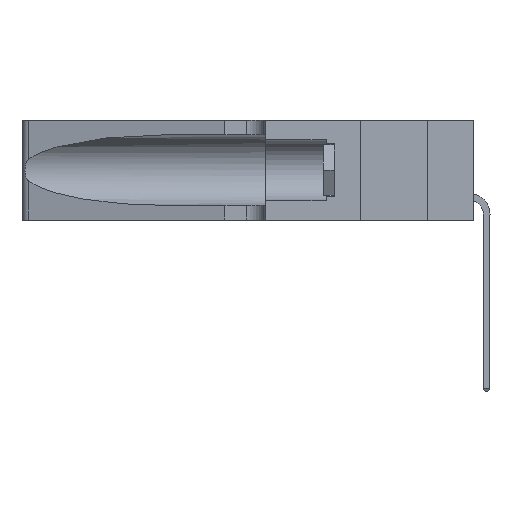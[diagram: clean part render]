
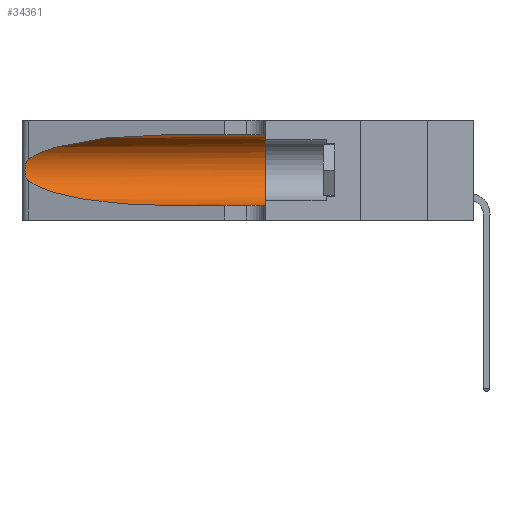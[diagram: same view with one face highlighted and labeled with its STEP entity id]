
A CAD part, left-side view. The second image highlights one B-rep face of the part: STEP entity #34361.
In plain terms, the highlighted cylindrical face has radius 3.308 mm (diameter 6.617 mm), a partial arc.
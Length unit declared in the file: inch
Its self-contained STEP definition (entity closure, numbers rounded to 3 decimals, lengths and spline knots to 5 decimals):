
#436 = CARTESIAN_POINT ( 'NONE',  ( 0.2373, 1.15595, 0.28018 ) ) ;
#444 =( BOUNDED_CURVE ( )  B_SPLINE_CURVE ( 3, ( #21980, #5683, #436, #24689 ),
 .UNSPECIFIED., .F., .F. ) 
 B_SPLINE_CURVE_WITH_KNOTS ( ( 4, 4 ),
 ( 1.5708, 2.84003 ),
 .UNSPECIFIED. ) 
 CURVE ( )  GEOMETRIC_REPRESENTATION_ITEM ( )  RATIONAL_B_SPLINE_CURVE ( ( 1., 0.87, 0.87, 1. ) ) 
 REPRESENTATION_ITEM ( '' )  );
#548 = ORIENTED_EDGE ( 'NONE', *, *, #11489, .F. ) ;
#1905 = CARTESIAN_POINT ( 'NONE',  ( 0.26018, 1.23835, 0.19895 ) ) ;
#3165 = VECTOR ( 'NONE', #34312, 39.37008 ) ;
#5121 = CARTESIAN_POINT ( 'NONE',  ( 0.25639, 1.23186, 0.15144 ) ) ;
#5570 = VERTEX_POINT ( 'NONE', #26565 ) ;
#5683 = CARTESIAN_POINT ( 'NONE',  ( 0.18966, 0.96281, 0.31525 ) ) ;
#6237 = CARTESIAN_POINT ( 'NONE',  ( 0.1305, 0.35, 0.31525 ) ) ;
#6379 = CARTESIAN_POINT ( 'NONE',  ( 0.18966, 0.96281, 0.05475 ) ) ;
#7819 = LINE ( 'NONE', #33601, #3165 ) ;
#7824 = EDGE_LOOP ( 'NONE', ( #22630, #31038, #19083, #35219, #32753, #548 ) ) ;
#8056 = CYLINDRICAL_SURFACE ( 'NONE', #14694, 0.13025 ) ;
#8565 = VERTEX_POINT ( 'NONE', #8575 ) ;
#8575 = CARTESIAN_POINT ( 'NONE',  ( 0.25487, 1.22718, 0.14631 ) ) ;
#8821 = VECTOR ( 'NONE', #16088, 39.37008 ) ;
#9594 = CARTESIAN_POINT ( 'NONE',  ( 0.1305, 1.61858, 0.185 ) ) ;
#10177 = CARTESIAN_POINT ( 'NONE',  ( 0.25856, 1.23593, 0.16098 ) ) ;
#10430 = CARTESIAN_POINT ( 'NONE',  ( 0.25639, 1.23184, 0.21858 ) ) ;
#11489 = EDGE_CURVE ( 'NONE', #34759, #23231, #7819, .T. ) ;
#13201 = CARTESIAN_POINT ( 'NONE',  ( 0.25789, 1.23486, 0.15765 ) ) ;
#13937 = CARTESIAN_POINT ( 'NONE',  ( 0.1305, 0.35, 0.185 ) ) ;
#14694 = AXIS2_PLACEMENT_3D ( 'NONE', #9594, #32220, #34705 ) ;
#15579 = CARTESIAN_POINT ( 'NONE',  ( 0.25555, 1.22994, 0.2215 ) ) ;
#15807 = CARTESIAN_POINT ( 'NONE',  ( 0.25487, 1.22718, 0.22369 ) ) ;
#16088 = DIRECTION ( 'NONE',  ( 0., -1., 0. ) ) ;
#16789 = B_SPLINE_CURVE_WITH_KNOTS ( 'NONE', 3,
 ( #15807, #15579, #10430, #21057, #34464, #1905, #34579, #34823, #26507, #10177, #13201, #5121, #18661, #29586 ),
 .UNSPECIFIED., .F., .F.,
 ( 4, 2, 2, 2, 2, 2, 4 ),
 ( 0., 0.00027, 0.00053, 0.00107, 0.0016, 0.00187, 0.00214 ),
 .UNSPECIFIED. ) ;
#17370 = EDGE_CURVE ( 'NONE', #23231, #27558, #29145, .T. ) ;
#17856 = AXIS2_PLACEMENT_3D ( 'NONE', #13937, #19528, #27142 ) ;
#18001 = EDGE_CURVE ( 'NONE', #34759, #31882, #444, .T. ) ;
#18661 = CARTESIAN_POINT ( 'NONE',  ( 0.25555, 1.22993, 0.14849 ) ) ;
#19083 = ORIENTED_EDGE ( 'NONE', *, *, #32806, .T. ) ;
#19177 = CARTESIAN_POINT ( 'NONE',  ( 0.1305, 0.35, 0.05475 ) ) ;
#19528 = DIRECTION ( 'NONE',  ( 0., 1., 0. ) ) ;
#19841 = CARTESIAN_POINT ( 'NONE',  ( 0.1305, 0.72297, 0.05475 ) ) ;
#21057 = CARTESIAN_POINT ( 'NONE',  ( 0.25787, 1.23484, 0.2124 ) ) ;
#21861 = CARTESIAN_POINT ( 'NONE',  ( 0.2373, 1.15595, 0.08982 ) ) ;
#21980 = CARTESIAN_POINT ( 'NONE',  ( 0.1305, 0.72297, 0.31525 ) ) ;
#22630 = ORIENTED_EDGE ( 'NONE', *, *, #18001, .T. ) ;
#23231 = VERTEX_POINT ( 'NONE', #6237 ) ;
#24115 = EDGE_CURVE ( 'NONE', #31882, #8565, #16789, .T. ) ;
#24276 = CARTESIAN_POINT ( 'NONE',  ( 0.1305, 1.61858, 0.05475 ) ) ;
#24689 = CARTESIAN_POINT ( 'NONE',  ( 0.25487, 1.22718, 0.22369 ) ) ;
#26507 = CARTESIAN_POINT ( 'NONE',  ( 0.26017, 1.23833, 0.17102 ) ) ;
#26565 = CARTESIAN_POINT ( 'NONE',  ( 0.1305, 0.72297, 0.05475 ) ) ;
#27142 = DIRECTION ( 'NONE',  ( 0., 0., 1. ) ) ;
#27558 = VERTEX_POINT ( 'NONE', #19177 ) ;
#28815 =( BOUNDED_CURVE ( )  B_SPLINE_CURVE ( 3, ( #32895, #21861, #6379, #19841 ),
 .UNSPECIFIED., .F., .T. ) 
 B_SPLINE_CURVE_WITH_KNOTS ( ( 4, 4 ),
 ( 3.44316, 4.71239 ),
 .UNSPECIFIED. ) 
 CURVE ( )  GEOMETRIC_REPRESENTATION_ITEM ( )  RATIONAL_B_SPLINE_CURVE ( ( 1., 0.87, 0.87, 1. ) ) 
 REPRESENTATION_ITEM ( '' )  );
#28826 = CARTESIAN_POINT ( 'NONE',  ( 0.1305, 0.72297, 0.31525 ) ) ;
#29145 = CIRCLE ( 'NONE', #17856, 0.13025 ) ;
#29586 = CARTESIAN_POINT ( 'NONE',  ( 0.25487, 1.22718, 0.14631 ) ) ;
#29642 = EDGE_CURVE ( 'NONE', #5570, #27558, #33504, .T. ) ;
#31038 = ORIENTED_EDGE ( 'NONE', *, *, #24115, .T. ) ;
#31882 = VERTEX_POINT ( 'NONE', #32140 ) ;
#32140 = CARTESIAN_POINT ( 'NONE',  ( 0.25487, 1.22718, 0.22369 ) ) ;
#32220 = DIRECTION ( 'NONE',  ( 0., -1., 0. ) ) ;
#32364 = FACE_OUTER_BOUND ( 'NONE', #7824, .T. ) ;
#32753 = ORIENTED_EDGE ( 'NONE', *, *, #17370, .F. ) ;
#32806 = EDGE_CURVE ( 'NONE', #8565, #5570, #28815, .T. ) ;
#32895 = CARTESIAN_POINT ( 'NONE',  ( 0.25487, 1.22718, 0.14631 ) ) ;
#33504 = LINE ( 'NONE', #24276, #8821 ) ;
#33601 = CARTESIAN_POINT ( 'NONE',  ( 0.1305, 1.61858, 0.31525 ) ) ;
#34312 = DIRECTION ( 'NONE',  ( 0., -1., 0. ) ) ;
#34361 = ADVANCED_FACE ( 'NONE', ( #32364 ), #8056, .F. ) ;
#34464 = CARTESIAN_POINT ( 'NONE',  ( 0.25854, 1.2359, 0.20912 ) ) ;
#34579 = CARTESIAN_POINT ( 'NONE',  ( 0.26075, 1.23896, 0.19203 ) ) ;
#34705 = DIRECTION ( 'NONE',  ( 0., 0., -1. ) ) ;
#34759 = VERTEX_POINT ( 'NONE', #28826 ) ;
#34823 = CARTESIAN_POINT ( 'NONE',  ( 0.26075, 1.23896, 0.178 ) ) ;
#35219 = ORIENTED_EDGE ( 'NONE', *, *, #29642, .T. ) ;
